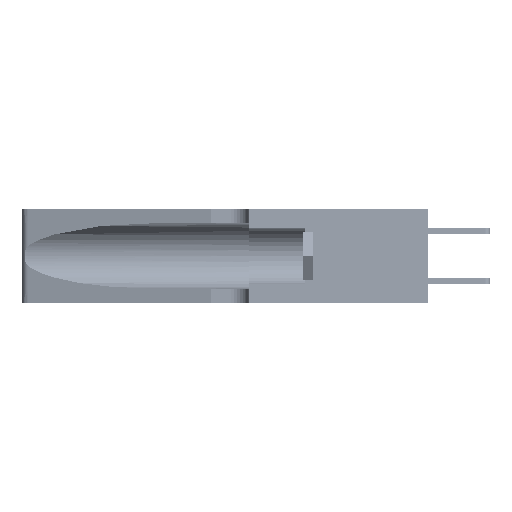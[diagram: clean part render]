
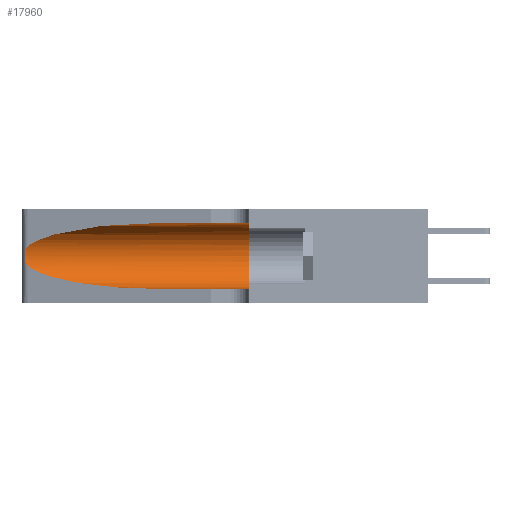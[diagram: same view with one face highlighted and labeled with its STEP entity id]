
A CAD part, left-side view. The second image highlights one B-rep face of the part: STEP entity #17960.
In plain terms, the highlighted cylindrical face has radius 3.308 mm (diameter 6.617 mm), a partial arc.
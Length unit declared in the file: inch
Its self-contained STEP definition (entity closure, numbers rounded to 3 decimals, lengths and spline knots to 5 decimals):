
#56 = CARTESIAN_POINT ( 'NONE',  ( 0.1305, 0.35, 0.185 ) ) ;
#217 = ORIENTED_EDGE ( 'NONE', *, *, #16272, .T. ) ;
#1315 =( BOUNDED_CURVE ( )  B_SPLINE_CURVE ( 3, ( #26300, #34451, #34279, #3129 ),
 .UNSPECIFIED., .F., .F. ) 
 B_SPLINE_CURVE_WITH_KNOTS ( ( 4, 4 ),
 ( 3.44316, 4.71239 ),
 .UNSPECIFIED. ) 
 CURVE ( )  GEOMETRIC_REPRESENTATION_ITEM ( )  RATIONAL_B_SPLINE_CURVE ( ( 1., 0.87, 0.87, 1. ) ) 
 REPRESENTATION_ITEM ( '' )  );
#2356 = CARTESIAN_POINT ( 'NONE',  ( 0.25854, 1.2359, 0.20912 ) ) ;
#2456 = DIRECTION ( 'NONE',  ( 0., 0., -1. ) ) ;
#3129 = CARTESIAN_POINT ( 'NONE',  ( 0.1305, 0.72297, 0.05475 ) ) ;
#3530 = CYLINDRICAL_SURFACE ( 'NONE', #22535, 0.13025 ) ;
#4177 = CARTESIAN_POINT ( 'NONE',  ( 0.1305, 0.72297, 0.05475 ) ) ;
#5117 = CARTESIAN_POINT ( 'NONE',  ( 0.1305, 1.61858, 0.05475 ) ) ;
#6155 = EDGE_CURVE ( 'NONE', #40413, #33561, #49312, .T. ) ;
#6419 = CARTESIAN_POINT ( 'NONE',  ( 0.25639, 1.23184, 0.21858 ) ) ;
#9765 = CARTESIAN_POINT ( 'NONE',  ( 0.2373, 1.15595, 0.28018 ) ) ;
#9803 = ORIENTED_EDGE ( 'NONE', *, *, #12011, .T. ) ;
#9997 = CARTESIAN_POINT ( 'NONE',  ( 0.26075, 1.23896, 0.178 ) ) ;
#10232 = CARTESIAN_POINT ( 'NONE',  ( 0.1305, 0.35, 0.31525 ) ) ;
#10305 = B_SPLINE_CURVE_WITH_KNOTS ( 'NONE', 3,
 ( #44485, #13552, #6419, #14059, #2356, #36904, #48224, #9997, #44312, #21307, #25056, #33344, #40600, #33509 ),
 .UNSPECIFIED., .F., .F.,
 ( 4, 2, 2, 2, 2, 2, 4 ),
 ( 0., 0.00027, 0.00053, 0.00107, 0.0016, 0.00187, 0.00214 ),
 .UNSPECIFIED. ) ;
#12011 = EDGE_CURVE ( 'NONE', #14819, #33561, #40545, .T. ) ;
#12108 = ORIENTED_EDGE ( 'NONE', *, *, #6155, .F. ) ;
#13138 = CARTESIAN_POINT ( 'NONE',  ( 0.18966, 0.96281, 0.31525 ) ) ;
#13552 = CARTESIAN_POINT ( 'NONE',  ( 0.25555, 1.22994, 0.2215 ) ) ;
#14059 = CARTESIAN_POINT ( 'NONE',  ( 0.25787, 1.23484, 0.2124 ) ) ;
#14819 = VERTEX_POINT ( 'NONE', #4177 ) ;
#15755 = CARTESIAN_POINT ( 'NONE',  ( 0.1305, 0.72297, 0.31525 ) ) ;
#15996 = CARTESIAN_POINT ( 'NONE',  ( 0.25487, 1.22718, 0.14631 ) ) ;
#16272 = EDGE_CURVE ( 'NONE', #44825, #49678, #10305, .T. ) ;
#17207 = ORIENTED_EDGE ( 'NONE', *, *, #17242, .T. ) ;
#17242 = EDGE_CURVE ( 'NONE', #49678, #14819, #1315, .T. ) ;
#17960 = ADVANCED_FACE ( 'NONE', ( #18059 ), #3530, .F. ) ;
#18059 = FACE_OUTER_BOUND ( 'NONE', #28517, .T. ) ;
#18166 = VECTOR ( 'NONE', #39475, 39.37008 ) ;
#21250 = CARTESIAN_POINT ( 'NONE',  ( 0.1305, 1.61858, 0.185 ) ) ;
#21307 = CARTESIAN_POINT ( 'NONE',  ( 0.25856, 1.23593, 0.16098 ) ) ;
#22535 = AXIS2_PLACEMENT_3D ( 'NONE', #21250, #44424, #2456 ) ;
#23011 =( BOUNDED_CURVE ( )  B_SPLINE_CURVE ( 3, ( #44587, #13138, #9765, #47985 ),
 .UNSPECIFIED., .F., .T. ) 
 B_SPLINE_CURVE_WITH_KNOTS ( ( 4, 4 ),
 ( 1.5708, 2.84003 ),
 .UNSPECIFIED. ) 
 CURVE ( )  GEOMETRIC_REPRESENTATION_ITEM ( )  RATIONAL_B_SPLINE_CURVE ( ( 1., 0.87, 0.87, 1. ) ) 
 REPRESENTATION_ITEM ( '' )  );
#24068 = ORIENTED_EDGE ( 'NONE', *, *, #47491, .F. ) ;
#24385 = CARTESIAN_POINT ( 'NONE',  ( 0.1305, 1.61858, 0.31525 ) ) ;
#25056 = CARTESIAN_POINT ( 'NONE',  ( 0.25789, 1.23486, 0.15765 ) ) ;
#26300 = CARTESIAN_POINT ( 'NONE',  ( 0.25487, 1.22718, 0.14631 ) ) ;
#27117 = CARTESIAN_POINT ( 'NONE',  ( 0.1305, 0.35, 0.05475 ) ) ;
#28517 = EDGE_LOOP ( 'NONE', ( #43788, #217, #17207, #9803, #12108, #24068 ) ) ;
#33344 = CARTESIAN_POINT ( 'NONE',  ( 0.25639, 1.23186, 0.15144 ) ) ;
#33509 = CARTESIAN_POINT ( 'NONE',  ( 0.25487, 1.22718, 0.14631 ) ) ;
#33561 = VERTEX_POINT ( 'NONE', #27117 ) ;
#34279 = CARTESIAN_POINT ( 'NONE',  ( 0.18966, 0.96281, 0.05475 ) ) ;
#34451 = CARTESIAN_POINT ( 'NONE',  ( 0.2373, 1.15595, 0.08982 ) ) ;
#34952 = DIRECTION ( 'NONE',  ( 0., 1., 0. ) ) ;
#36904 = CARTESIAN_POINT ( 'NONE',  ( 0.26018, 1.23835, 0.19895 ) ) ;
#37742 = LINE ( 'NONE', #24385, #44392 ) ;
#38786 = EDGE_CURVE ( 'NONE', #43916, #44825, #23011, .T. ) ;
#39475 = DIRECTION ( 'NONE',  ( 0., -1., 0. ) ) ;
#40413 = VERTEX_POINT ( 'NONE', #10232 ) ;
#40545 = LINE ( 'NONE', #5117, #18166 ) ;
#40600 = CARTESIAN_POINT ( 'NONE',  ( 0.25555, 1.22993, 0.14849 ) ) ;
#42702 = DIRECTION ( 'NONE',  ( 0., 0., 1. ) ) ;
#43788 = ORIENTED_EDGE ( 'NONE', *, *, #38786, .T. ) ;
#43916 = VERTEX_POINT ( 'NONE', #15755 ) ;
#44311 = DIRECTION ( 'NONE',  ( 0., -1., 0. ) ) ;
#44312 = CARTESIAN_POINT ( 'NONE',  ( 0.26017, 1.23833, 0.17102 ) ) ;
#44392 = VECTOR ( 'NONE', #44311, 39.37008 ) ;
#44424 = DIRECTION ( 'NONE',  ( 0., -1., 0. ) ) ;
#44485 = CARTESIAN_POINT ( 'NONE',  ( 0.25487, 1.22718, 0.22369 ) ) ;
#44587 = CARTESIAN_POINT ( 'NONE',  ( 0.1305, 0.72297, 0.31525 ) ) ;
#44825 = VERTEX_POINT ( 'NONE', #48347 ) ;
#47491 = EDGE_CURVE ( 'NONE', #43916, #40413, #37742, .T. ) ;
#47568 = AXIS2_PLACEMENT_3D ( 'NONE', #56, #34952, #42702 ) ;
#47985 = CARTESIAN_POINT ( 'NONE',  ( 0.25487, 1.22718, 0.22369 ) ) ;
#48224 = CARTESIAN_POINT ( 'NONE',  ( 0.26075, 1.23896, 0.19203 ) ) ;
#48347 = CARTESIAN_POINT ( 'NONE',  ( 0.25487, 1.22718, 0.22369 ) ) ;
#49312 = CIRCLE ( 'NONE', #47568, 0.13025 ) ;
#49678 = VERTEX_POINT ( 'NONE', #15996 ) ;
